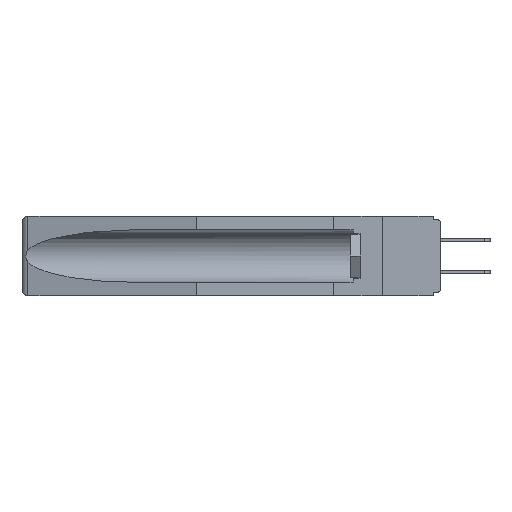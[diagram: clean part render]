
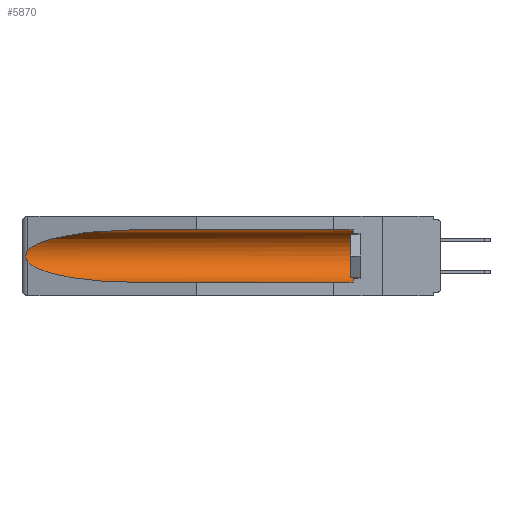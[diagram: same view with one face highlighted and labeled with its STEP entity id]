
A CAD part, left-side view. The second image highlights one B-rep face of the part: STEP entity #5870.
In plain terms, the highlighted cylindrical face has radius 2.857 mm (diameter 5.715 mm), a partial arc.
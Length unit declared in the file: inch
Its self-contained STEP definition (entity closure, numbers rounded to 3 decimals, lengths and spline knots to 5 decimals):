
#990 = EDGE_CURVE ( 'NONE', #1470, #24950, #9615, .T. ) ;
#1173 = CARTESIAN_POINT ( 'NONE',  ( 0.155, -0.30754, -0.1715 ) ) ;
#1386 = CARTESIAN_POINT ( 'NONE',  ( 0.155, 0.126, -0.284 ) ) ;
#1425 = CARTESIAN_POINT ( 'NONE',  ( 0.26597, 1.5296, -0.19026 ) ) ;
#1470 = VERTEX_POINT ( 'NONE', #1386 ) ;
#2781 = EDGE_CURVE ( 'NONE', #12381, #24950, #9581, .T. ) ;
#2905 = DIRECTION ( 'NONE',  ( 0., 0., 1. ) ) ;
#3058 = ORIENTED_EDGE ( 'NONE', *, *, #23812, .T. ) ;
#3102 = AXIS2_PLACEMENT_3D ( 'NONE', #19676, #9616, #5665 ) ;
#3430 = CARTESIAN_POINT ( 'NONE',  ( 0.26655, 1.53094, -0.18657 ) ) ;
#4537 = EDGE_CURVE ( 'NONE', #5210, #21999, #7441, .T. ) ;
#4675 = CARTESIAN_POINT ( 'NONE',  ( 0.26537, 1.52718, -0.19328 ) ) ;
#4721 = CARTESIAN_POINT ( 'NONE',  ( 0.26537, 1.52718, -0.14972 ) ) ;
#4928 = CARTESIAN_POINT ( 'NONE',  ( 0.155, -0.30754, -0.284 ) ) ;
#5210 = VERTEX_POINT ( 'NONE', #18351 ) ;
#5364 = CARTESIAN_POINT ( 'NONE',  ( 0.26537, 1.52718, -0.14972 ) ) ;
#5445 = CARTESIAN_POINT ( 'NONE',  ( 0.2675, 1.53308, -0.17534 ) ) ;
#5661 = DIRECTION ( 'NONE',  ( 0., 1., 0. ) ) ;
#5665 = DIRECTION ( 'NONE',  ( 0., 0., 1. ) ) ;
#5686 = CARTESIAN_POINT ( 'NONE',  ( 0.26537, 1.52718, -0.14972 ) ) ;
#5870 = ADVANCED_FACE ( 'NONE', ( #24768 ), #7360, .F. ) ;
#7360 = CYLINDRICAL_SURFACE ( 'NONE', #23262, 0.1125 ) ;
#7441 = LINE ( 'NONE', #25017, #13310 ) ;
#7698 = ORIENTED_EDGE ( 'NONE', *, *, #4537, .T. ) ;
#8345 = CARTESIAN_POINT ( 'NONE',  ( 0.155, 1.07973, -0.059 ) ) ;
#9240 = CARTESIAN_POINT ( 'NONE',  ( 0.155, 1.07973, -0.284 ) ) ;
#9250 = ORIENTED_EDGE ( 'NONE', *, *, #2781, .T. ) ;
#9581 =( BOUNDED_CURVE ( )  B_SPLINE_CURVE ( 3, ( #17217, #17125, #22986, #9240 ),
 .UNSPECIFIED., .F., .F. ) 
 B_SPLINE_CURVE_WITH_KNOTS ( ( 4, 4 ),
 ( 0.1948, 1.5708 ),
 .UNSPECIFIED. ) 
 CURVE ( )  GEOMETRIC_REPRESENTATION_ITEM ( )  RATIONAL_B_SPLINE_CURVE ( ( 1., 0.848, 0.848, 1. ) ) 
 REPRESENTATION_ITEM ( '' )  );
#9615 = LINE ( 'NONE', #4928, #23635 ) ;
#9616 = DIRECTION ( 'NONE',  ( 0., -1., 0. ) ) ;
#11199 = CARTESIAN_POINT ( 'NONE',  ( 0.26537, 1.52718, -0.19328 ) ) ;
#11449 = CARTESIAN_POINT ( 'NONE',  ( 0.155, 1.07973, -0.059 ) ) ;
#11785 = EDGE_LOOP ( 'NONE', ( #22244, #3058, #9250, #24188, #14573, #7698 ) ) ;
#12381 = VERTEX_POINT ( 'NONE', #4675 ) ;
#12936 = EDGE_CURVE ( 'NONE', #1470, #5210, #23520, .T. ) ;
#13310 = VECTOR ( 'NONE', #17171, 39.37008 ) ;
#14573 = ORIENTED_EDGE ( 'NONE', *, *, #12936, .T. ) ;
#15257 = CARTESIAN_POINT ( 'NONE',  ( 0.155, 1.07973, -0.284 ) ) ;
#15443 = CARTESIAN_POINT ( 'NONE',  ( 0.26597, 1.52961, -0.15275 ) ) ;
#15511 = CARTESIAN_POINT ( 'NONE',  ( 0.21114, 1.30732, -0.059 ) ) ;
#15773 = B_SPLINE_CURVE_WITH_KNOTS ( 'NONE', 3,
 ( #5364, #15443, #23401, #21474, #23132, #5445, #19270, #3430, #1425, #11199 ),
 .UNSPECIFIED., .F., .F.,
 ( 4, 2, 2, 2, 4 ),
 ( 0., 0.00029, 0.00058, 0.00087, 0.00117 ),
 .UNSPECIFIED. ) ;
#16780 = DIRECTION ( 'NONE',  ( 0., 1., 0. ) ) ;
#17125 = CARTESIAN_POINT ( 'NONE',  ( 0.25451, 1.48313, -0.24835 ) ) ;
#17171 = DIRECTION ( 'NONE',  ( 0., 1., 0. ) ) ;
#17217 = CARTESIAN_POINT ( 'NONE',  ( 0.26537, 1.52718, -0.19328 ) ) ;
#17534 = CARTESIAN_POINT ( 'NONE',  ( 0.25451, 1.48313, -0.09465 ) ) ;
#18351 = CARTESIAN_POINT ( 'NONE',  ( 0.155, 0.126, -0.059 ) ) ;
#19270 = CARTESIAN_POINT ( 'NONE',  ( 0.2673, 1.53269, -0.17917 ) ) ;
#19676 = CARTESIAN_POINT ( 'NONE',  ( 0.155, 0.126, -0.1715 ) ) ;
#20616 = EDGE_CURVE ( 'NONE', #21999, #22799, #25022, .T. ) ;
#21474 = CARTESIAN_POINT ( 'NONE',  ( 0.2673, 1.5327, -0.16383 ) ) ;
#21999 = VERTEX_POINT ( 'NONE', #8345 ) ;
#22244 = ORIENTED_EDGE ( 'NONE', *, *, #20616, .T. ) ;
#22799 = VERTEX_POINT ( 'NONE', #4721 ) ;
#22986 = CARTESIAN_POINT ( 'NONE',  ( 0.21114, 1.30732, -0.284 ) ) ;
#23132 = CARTESIAN_POINT ( 'NONE',  ( 0.2675, 1.53308, -0.16763 ) ) ;
#23262 = AXIS2_PLACEMENT_3D ( 'NONE', #1173, #16780, #2905 ) ;
#23401 = CARTESIAN_POINT ( 'NONE',  ( 0.26654, 1.53092, -0.15636 ) ) ;
#23520 = CIRCLE ( 'NONE', #3102, 0.1125 ) ;
#23635 = VECTOR ( 'NONE', #5661, 39.37008 ) ;
#23812 = EDGE_CURVE ( 'NONE', #22799, #12381, #15773, .T. ) ;
#24188 = ORIENTED_EDGE ( 'NONE', *, *, #990, .F. ) ;
#24768 = FACE_OUTER_BOUND ( 'NONE', #11785, .T. ) ;
#24950 = VERTEX_POINT ( 'NONE', #15257 ) ;
#25017 = CARTESIAN_POINT ( 'NONE',  ( 0.155, -0.30754, -0.059 ) ) ;
#25022 =( BOUNDED_CURVE ( )  B_SPLINE_CURVE ( 3, ( #11449, #15511, #17534, #5686 ),
 .UNSPECIFIED., .F., .F. ) 
 B_SPLINE_CURVE_WITH_KNOTS ( ( 4, 4 ),
 ( 4.71239, 6.08839 ),
 .UNSPECIFIED. ) 
 CURVE ( )  GEOMETRIC_REPRESENTATION_ITEM ( )  RATIONAL_B_SPLINE_CURVE ( ( 1., 0.848, 0.848, 1. ) ) 
 REPRESENTATION_ITEM ( '' )  );
